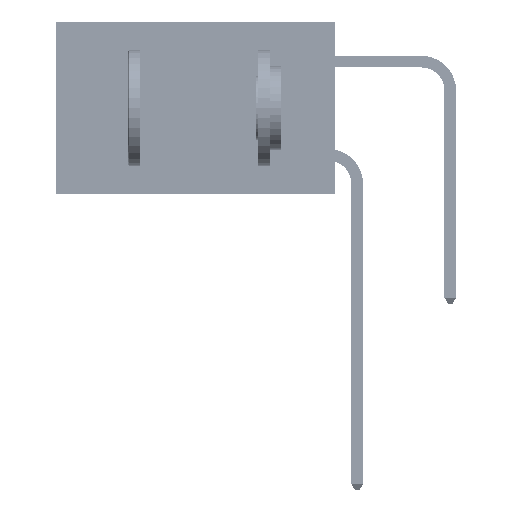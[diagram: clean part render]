
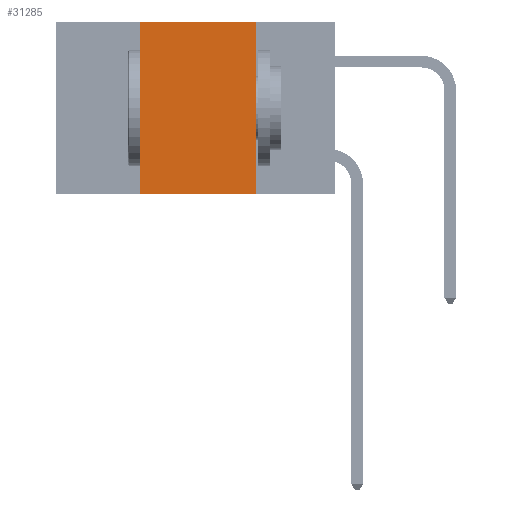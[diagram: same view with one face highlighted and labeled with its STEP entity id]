
A CAD part, left-side view. The second image highlights one B-rep face of the part: STEP entity #31285.
In plain terms, the highlighted planar face has unit normal (-1, 0, 0).
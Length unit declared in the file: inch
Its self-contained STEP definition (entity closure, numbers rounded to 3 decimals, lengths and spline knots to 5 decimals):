
#2183 = ORIENTED_EDGE ( 'NONE', *, *, #16541, .T. ) ;
#3433 = VECTOR ( 'NONE', #4768, 39.37008 ) ;
#4768 = DIRECTION ( 'NONE',  ( 0., 0., -1. ) ) ;
#6042 = CARTESIAN_POINT ( 'NONE',  ( 0., 0.6, 0. ) ) ;
#6114 = CARTESIAN_POINT ( 'NONE',  ( 0., 0.6, -0.37 ) ) ;
#6741 = LINE ( 'NONE', #30136, #3433 ) ;
#7487 = DIRECTION ( 'NONE',  ( 0., -1., 0. ) ) ;
#8965 = VERTEX_POINT ( 'NONE', #15988 ) ;
#9575 = DIRECTION ( 'NONE',  ( 1., 0., 0. ) ) ;
#9813 = VECTOR ( 'NONE', #20553, 39.37008 ) ;
#11575 = VECTOR ( 'NONE', #35741, 39.37008 ) ;
#15988 = CARTESIAN_POINT ( 'NONE',  ( 0., 0.42, 0. ) ) ;
#16541 = EDGE_CURVE ( 'NONE', #50906, #29822, #21545, .T. ) ;
#19358 = CARTESIAN_POINT ( 'NONE',  ( 0., 0.17, 0. ) ) ;
#20289 = LINE ( 'NONE', #28938, #47441 ) ;
#20553 = DIRECTION ( 'NONE',  ( 0., 0., 1. ) ) ;
#21545 = LINE ( 'NONE', #6114, #11575 ) ;
#23260 = FACE_OUTER_BOUND ( 'NONE', #24972, .T. ) ;
#24972 = EDGE_LOOP ( 'NONE', ( #54744, #29489, #29439, #2183 ) ) ;
#25513 = CARTESIAN_POINT ( 'NONE',  ( 0., 0.42, 0. ) ) ;
#27728 = EDGE_CURVE ( 'NONE', #8965, #40319, #20289, .T. ) ;
#28938 = CARTESIAN_POINT ( 'NONE',  ( 0., 0.6, 0. ) ) ;
#29439 = ORIENTED_EDGE ( 'NONE', *, *, #54793, .F. ) ;
#29489 = ORIENTED_EDGE ( 'NONE', *, *, #27728, .F. ) ;
#29822 = VERTEX_POINT ( 'NONE', #34532 ) ;
#30136 = CARTESIAN_POINT ( 'NONE',  ( 0., 0.17, 0. ) ) ;
#31285 = ADVANCED_FACE ( 'NONE', ( #23260 ), #35675, .F. ) ;
#34402 = EDGE_CURVE ( 'NONE', #40319, #29822, #6741, .T. ) ;
#34532 = CARTESIAN_POINT ( 'NONE',  ( 0., 0.17, -0.37 ) ) ;
#35675 = PLANE ( 'NONE',  #46654 ) ;
#35741 = DIRECTION ( 'NONE',  ( 0., -1., 0. ) ) ;
#38969 = LINE ( 'NONE', #25513, #9813 ) ;
#40319 = VERTEX_POINT ( 'NONE', #19358 ) ;
#43629 = DIRECTION ( 'NONE',  ( 0., 0., -1. ) ) ;
#45625 = CARTESIAN_POINT ( 'NONE',  ( 0., 0.42, -0.37 ) ) ;
#46654 = AXIS2_PLACEMENT_3D ( 'NONE', #6042, #9575, #43629 ) ;
#47441 = VECTOR ( 'NONE', #7487, 39.37008 ) ;
#50906 = VERTEX_POINT ( 'NONE', #45625 ) ;
#54744 = ORIENTED_EDGE ( 'NONE', *, *, #34402, .F. ) ;
#54793 = EDGE_CURVE ( 'NONE', #50906, #8965, #38969, .T. ) ;
